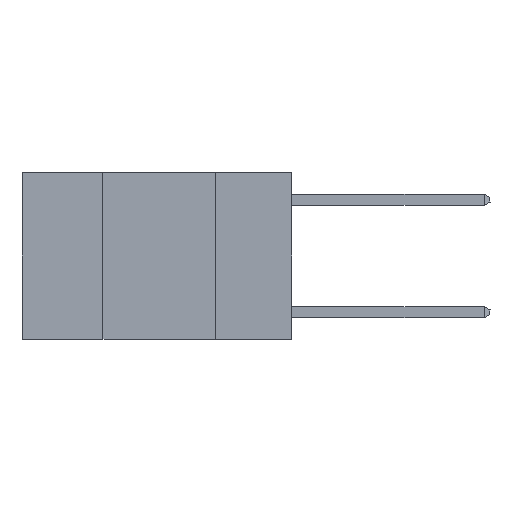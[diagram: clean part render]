
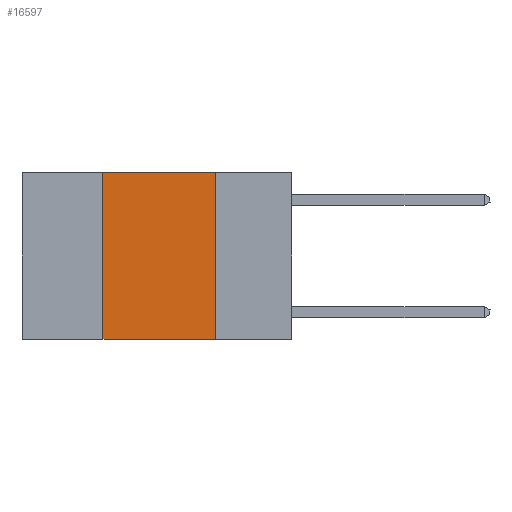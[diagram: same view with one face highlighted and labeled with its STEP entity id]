
A CAD part, left-side view. The second image highlights one B-rep face of the part: STEP entity #16597.
In plain terms, the highlighted planar face has unit normal (-1, 0, 0).
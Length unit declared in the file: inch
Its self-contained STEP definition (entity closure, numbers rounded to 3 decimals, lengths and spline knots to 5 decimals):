
#1239 = VECTOR ( 'NONE', #4912, 39.37008 ) ;
#1459 = VECTOR ( 'NONE', #11961, 39.37008 ) ;
#1960 = DIRECTION ( 'NONE',  ( 0., 0., 1. ) ) ;
#2466 = LINE ( 'NONE', #15025, #1459 ) ;
#3426 = CARTESIAN_POINT ( 'NONE',  ( 0., 0.42, 0. ) ) ;
#3565 = CARTESIAN_POINT ( 'NONE',  ( 0., 0.17, 0. ) ) ;
#4405 = PLANE ( 'NONE',  #12397 ) ;
#4912 = DIRECTION ( 'NONE',  ( 0., -1., 0. ) ) ;
#5933 = DIRECTION ( 'NONE',  ( 0., 0., -1. ) ) ;
#6389 = CARTESIAN_POINT ( 'NONE',  ( 0., 0.42, -0.37 ) ) ;
#7071 = ORIENTED_EDGE ( 'NONE', *, *, #14421, .F. ) ;
#7868 = EDGE_CURVE ( 'NONE', #9650, #9686, #9513, .T. ) ;
#7915 = FACE_OUTER_BOUND ( 'NONE', #16947, .T. ) ;
#9513 = LINE ( 'NONE', #15659, #1239 ) ;
#9650 = VERTEX_POINT ( 'NONE', #3426 ) ;
#9686 = VERTEX_POINT ( 'NONE', #3565 ) ;
#10055 = ORIENTED_EDGE ( 'NONE', *, *, #7868, .F. ) ;
#10230 = VECTOR ( 'NONE', #1960, 39.37008 ) ;
#10755 = CARTESIAN_POINT ( 'NONE',  ( 0., 0.6, -0.37 ) ) ;
#10982 = LINE ( 'NONE', #10755, #15028 ) ;
#11961 = DIRECTION ( 'NONE',  ( 0., 0., -1. ) ) ;
#12397 = AXIS2_PLACEMENT_3D ( 'NONE', #19584, #15187, #5933 ) ;
#12817 = CARTESIAN_POINT ( 'NONE',  ( 0., 0.42, 0. ) ) ;
#12933 = ORIENTED_EDGE ( 'NONE', *, *, #14049, .F. ) ;
#12958 = VERTEX_POINT ( 'NONE', #6389 ) ;
#13894 = ORIENTED_EDGE ( 'NONE', *, *, #14171, .T. ) ;
#14049 = EDGE_CURVE ( 'NONE', #9686, #14428, #2466, .T. ) ;
#14171 = EDGE_CURVE ( 'NONE', #12958, #14428, #10982, .T. ) ;
#14338 = CARTESIAN_POINT ( 'NONE',  ( 0., 0.17, -0.37 ) ) ;
#14421 = EDGE_CURVE ( 'NONE', #12958, #9650, #18278, .T. ) ;
#14428 = VERTEX_POINT ( 'NONE', #14338 ) ;
#15025 = CARTESIAN_POINT ( 'NONE',  ( 0., 0.17, 0. ) ) ;
#15028 = VECTOR ( 'NONE', #18275, 39.37008 ) ;
#15187 = DIRECTION ( 'NONE',  ( 1., 0., 0. ) ) ;
#15659 = CARTESIAN_POINT ( 'NONE',  ( 0., 0.6, 0. ) ) ;
#16597 = ADVANCED_FACE ( 'NONE', ( #7915 ), #4405, .F. ) ;
#16947 = EDGE_LOOP ( 'NONE', ( #12933, #10055, #7071, #13894 ) ) ;
#18275 = DIRECTION ( 'NONE',  ( 0., -1., 0. ) ) ;
#18278 = LINE ( 'NONE', #12817, #10230 ) ;
#19584 = CARTESIAN_POINT ( 'NONE',  ( 0., 0.6, 0. ) ) ;
